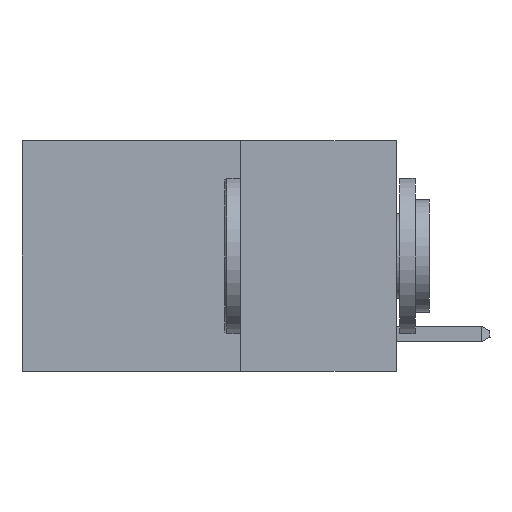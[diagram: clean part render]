
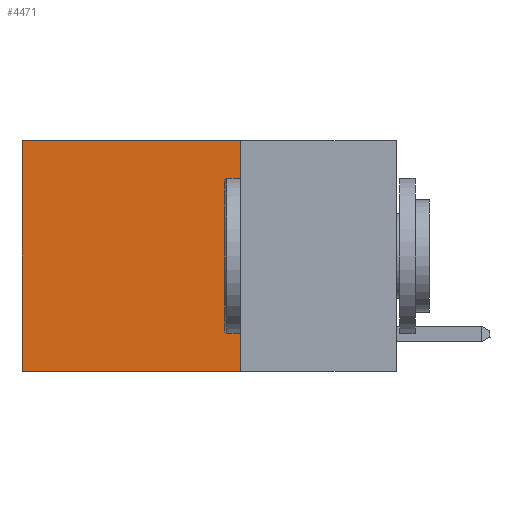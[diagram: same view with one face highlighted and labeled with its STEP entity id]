
A CAD part, left-side view. The second image highlights one B-rep face of the part: STEP entity #4471.
In plain terms, the highlighted planar face has unit normal (-1, 0, 0).
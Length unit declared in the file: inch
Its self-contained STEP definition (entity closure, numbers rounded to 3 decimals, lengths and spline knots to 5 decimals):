
#1148 = EDGE_CURVE ( 'NONE', #14605, #15417, #3438, .T. ) ;
#1598 = CARTESIAN_POINT ( 'NONE',  ( 0.2625, 0.6, 0. ) ) ;
#1895 = DIRECTION ( 'NONE',  ( 1., 0., 0. ) ) ;
#3438 = LINE ( 'NONE', #1598, #12717 ) ;
#3909 = LINE ( 'NONE', #20191, #22297 ) ;
#4471 = ADVANCED_FACE ( 'NONE', ( #12954 ), #13040, .F. ) ;
#5622 = CARTESIAN_POINT ( 'NONE',  ( 0.2625, 0.6, -0.37 ) ) ;
#7015 = CARTESIAN_POINT ( 'NONE',  ( 0.2625, 0.25, -0.37 ) ) ;
#7195 = CARTESIAN_POINT ( 'NONE',  ( 0.2625, 0.6, 0. ) ) ;
#7687 = ORIENTED_EDGE ( 'NONE', *, *, #1148, .T. ) ;
#8566 = AXIS2_PLACEMENT_3D ( 'NONE', #20287, #1895, #14892 ) ;
#9107 = ORIENTED_EDGE ( 'NONE', *, *, #11279, .F. ) ;
#10278 = CARTESIAN_POINT ( 'NONE',  ( 0.2625, 0.25, 0. ) ) ;
#10558 = ORIENTED_EDGE ( 'NONE', *, *, #23164, .F. ) ;
#10574 = ORIENTED_EDGE ( 'NONE', *, *, #12944, .T. ) ;
#10816 = CARTESIAN_POINT ( 'NONE',  ( 0.2625, 0.25, 0. ) ) ;
#11279 = EDGE_CURVE ( 'NONE', #13581, #15417, #16218, .T. ) ;
#12717 = VECTOR ( 'NONE', #23611, 39.37008 ) ;
#12944 = EDGE_CURVE ( 'NONE', #13785, #14605, #17003, .T. ) ;
#12954 = FACE_OUTER_BOUND ( 'NONE', #16562, .T. ) ;
#13040 = PLANE ( 'NONE',  #8566 ) ;
#13581 = VERTEX_POINT ( 'NONE', #22931 ) ;
#13785 = VERTEX_POINT ( 'NONE', #10816 ) ;
#14127 = VECTOR ( 'NONE', #15843, 39.37008 ) ;
#14605 = VERTEX_POINT ( 'NONE', #7195 ) ;
#14892 = DIRECTION ( 'NONE',  ( 0., 0., -1. ) ) ;
#15417 = VERTEX_POINT ( 'NONE', #5622 ) ;
#15843 = DIRECTION ( 'NONE',  ( 0., 1., 0. ) ) ;
#16218 = LINE ( 'NONE', #7015, #21026 ) ;
#16562 = EDGE_LOOP ( 'NONE', ( #7687, #9107, #10558, #10574 ) ) ;
#17003 = LINE ( 'NONE', #10278, #14127 ) ;
#19869 = DIRECTION ( 'NONE',  ( 0., 1., 0. ) ) ;
#20191 = CARTESIAN_POINT ( 'NONE',  ( 0.2625, 0.25, 0. ) ) ;
#20287 = CARTESIAN_POINT ( 'NONE',  ( 0.2625, 0.25, 0. ) ) ;
#21026 = VECTOR ( 'NONE', #19869, 39.37008 ) ;
#21998 = DIRECTION ( 'NONE',  ( 0., 0., -1. ) ) ;
#22297 = VECTOR ( 'NONE', #21998, 39.37008 ) ;
#22931 = CARTESIAN_POINT ( 'NONE',  ( 0.2625, 0.25, -0.37 ) ) ;
#23164 = EDGE_CURVE ( 'NONE', #13785, #13581, #3909, .T. ) ;
#23611 = DIRECTION ( 'NONE',  ( 0., 0., -1. ) ) ;
